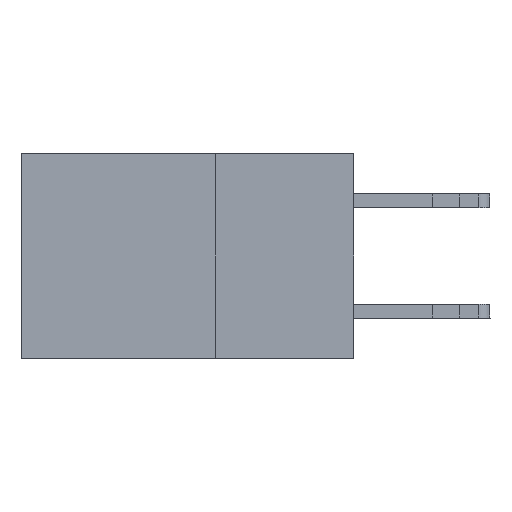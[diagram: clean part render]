
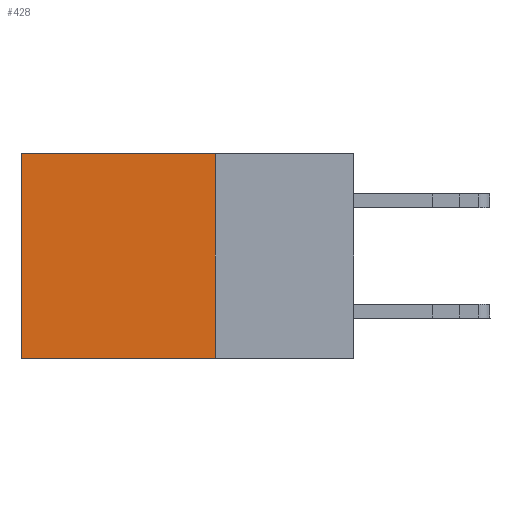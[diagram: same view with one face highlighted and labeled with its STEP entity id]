
A CAD part, left-side view. The second image highlights one B-rep face of the part: STEP entity #428.
In plain terms, the highlighted planar face has unit normal (-1, 0, 0).
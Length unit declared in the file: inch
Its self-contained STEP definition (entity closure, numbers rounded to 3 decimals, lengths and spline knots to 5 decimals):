
#67 = VECTOR ( 'NONE', #4622, 39.37008 ) ;
#118 = LINE ( 'NONE', #13448, #6828 ) ;
#428 = ADVANCED_FACE ( 'NONE', ( #1795 ), #17948, .F. ) ;
#1460 = AXIS2_PLACEMENT_3D ( 'NONE', #8285, #7953, #21477 ) ;
#1795 = FACE_OUTER_BOUND ( 'NONE', #2624, .T. ) ;
#2122 = EDGE_CURVE ( 'NONE', #16106, #11512, #118, .T. ) ;
#2624 = EDGE_LOOP ( 'NONE', ( #12239, #12345, #22820, #4077 ) ) ;
#4077 = ORIENTED_EDGE ( 'NONE', *, *, #6281, .T. ) ;
#4622 = DIRECTION ( 'NONE',  ( 0., 1., 0. ) ) ;
#5906 = EDGE_CURVE ( 'NONE', #10202, #17689, #12047, .T. ) ;
#6034 = CARTESIAN_POINT ( 'NONE',  ( 0.2875, 0.6, 0. ) ) ;
#6281 = EDGE_CURVE ( 'NONE', #16106, #10202, #17439, .T. ) ;
#6828 = VECTOR ( 'NONE', #22842, 39.37008 ) ;
#7195 = VECTOR ( 'NONE', #18801, 39.37008 ) ;
#7292 = CARTESIAN_POINT ( 'NONE',  ( 0.2875, 0.6, -0.37 ) ) ;
#7819 = VECTOR ( 'NONE', #13805, 39.37008 ) ;
#7953 = DIRECTION ( 'NONE',  ( 1., 0., 0. ) ) ;
#8285 = CARTESIAN_POINT ( 'NONE',  ( 0.2875, 0.25, 0. ) ) ;
#10202 = VERTEX_POINT ( 'NONE', #20813 ) ;
#11512 = VERTEX_POINT ( 'NONE', #22302 ) ;
#12047 = LINE ( 'NONE', #6034, #7819 ) ;
#12239 = ORIENTED_EDGE ( 'NONE', *, *, #5906, .T. ) ;
#12345 = ORIENTED_EDGE ( 'NONE', *, *, #22299, .F. ) ;
#12942 = CARTESIAN_POINT ( 'NONE',  ( 0.2875, 0.25, -0.37 ) ) ;
#13448 = CARTESIAN_POINT ( 'NONE',  ( 0.2875, 0.25, 0. ) ) ;
#13805 = DIRECTION ( 'NONE',  ( 0., 0., -1. ) ) ;
#16106 = VERTEX_POINT ( 'NONE', #21883 ) ;
#17439 = LINE ( 'NONE', #23687, #67 ) ;
#17689 = VERTEX_POINT ( 'NONE', #7292 ) ;
#17948 = PLANE ( 'NONE',  #1460 ) ;
#18801 = DIRECTION ( 'NONE',  ( 0., 1., 0. ) ) ;
#20813 = CARTESIAN_POINT ( 'NONE',  ( 0.2875, 0.6, 0. ) ) ;
#21477 = DIRECTION ( 'NONE',  ( 0., 0., -1. ) ) ;
#21883 = CARTESIAN_POINT ( 'NONE',  ( 0.2875, 0.25, 0. ) ) ;
#22299 = EDGE_CURVE ( 'NONE', #11512, #17689, #22629, .T. ) ;
#22302 = CARTESIAN_POINT ( 'NONE',  ( 0.2875, 0.25, -0.37 ) ) ;
#22629 = LINE ( 'NONE', #12942, #7195 ) ;
#22820 = ORIENTED_EDGE ( 'NONE', *, *, #2122, .F. ) ;
#22842 = DIRECTION ( 'NONE',  ( 0., 0., -1. ) ) ;
#23687 = CARTESIAN_POINT ( 'NONE',  ( 0.2875, 0.25, 0. ) ) ;
